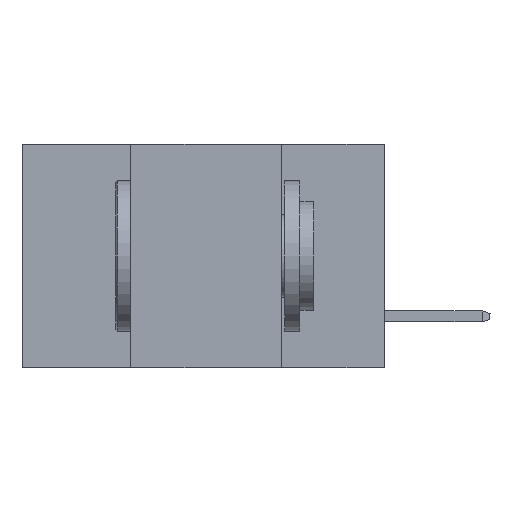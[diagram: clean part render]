
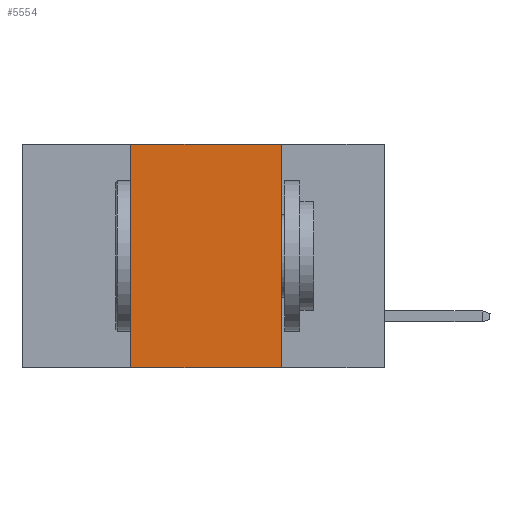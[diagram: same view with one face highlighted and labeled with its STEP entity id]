
A CAD part, left-side view. The second image highlights one B-rep face of the part: STEP entity #5554.
In plain terms, the highlighted planar face has unit normal (-1, 0, 0).
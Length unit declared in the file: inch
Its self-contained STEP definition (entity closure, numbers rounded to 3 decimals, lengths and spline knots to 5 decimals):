
#119 = CARTESIAN_POINT ( 'NONE',  ( 0., 0.17, 0. ) ) ;
#517 = VECTOR ( 'NONE', #2642, 39.37008 ) ;
#700 = DIRECTION ( 'NONE',  ( 0., -1., 0. ) ) ;
#762 = DIRECTION ( 'NONE',  ( 0., 0., -1. ) ) ;
#1027 = ORIENTED_EDGE ( 'NONE', *, *, #10004, .T. ) ;
#1449 = ORIENTED_EDGE ( 'NONE', *, *, #20818, .F. ) ;
#1867 = ORIENTED_EDGE ( 'NONE', *, *, #14197, .F. ) ;
#2285 = CARTESIAN_POINT ( 'NONE',  ( 0., 0.17, -0.37 ) ) ;
#2642 = DIRECTION ( 'NONE',  ( 0., 0., 1. ) ) ;
#2857 = LINE ( 'NONE', #10920, #517 ) ;
#3102 = VECTOR ( 'NONE', #15820, 39.37008 ) ;
#3290 = VERTEX_POINT ( 'NONE', #2285 ) ;
#3580 = DIRECTION ( 'NONE',  ( 1., 0., 0. ) ) ;
#4386 = VECTOR ( 'NONE', #700, 39.37008 ) ;
#5554 = ADVANCED_FACE ( 'NONE', ( #11743 ), #20213, .F. ) ;
#7330 = CARTESIAN_POINT ( 'NONE',  ( 0., 0.6, -0.37 ) ) ;
#8270 = EDGE_CURVE ( 'NONE', #14796, #3290, #19157, .T. ) ;
#9048 = LINE ( 'NONE', #7330, #18968 ) ;
#10004 = EDGE_CURVE ( 'NONE', #20821, #3290, #9048, .T. ) ;
#10497 = LINE ( 'NONE', #15432, #4386 ) ;
#10625 = CARTESIAN_POINT ( 'NONE',  ( 0., 0.42, 0. ) ) ;
#10920 = CARTESIAN_POINT ( 'NONE',  ( 0., 0.42, -0.37 ) ) ;
#11743 = FACE_OUTER_BOUND ( 'NONE', #13374, .T. ) ;
#11951 = AXIS2_PLACEMENT_3D ( 'NONE', #18276, #3580, #762 ) ;
#12623 = CARTESIAN_POINT ( 'NONE',  ( 0., 0.42, -0.37 ) ) ;
#13374 = EDGE_LOOP ( 'NONE', ( #16656, #1867, #1449, #1027 ) ) ;
#13596 = VERTEX_POINT ( 'NONE', #10625 ) ;
#14197 = EDGE_CURVE ( 'NONE', #13596, #14796, #10497, .T. ) ;
#14796 = VERTEX_POINT ( 'NONE', #119 ) ;
#15432 = CARTESIAN_POINT ( 'NONE',  ( 0., 0.6, 0. ) ) ;
#15820 = DIRECTION ( 'NONE',  ( 0., 0., -1. ) ) ;
#16656 = ORIENTED_EDGE ( 'NONE', *, *, #8270, .F. ) ;
#17731 = CARTESIAN_POINT ( 'NONE',  ( 0., 0.17, -0.37 ) ) ;
#18276 = CARTESIAN_POINT ( 'NONE',  ( 0., 0.6, 0. ) ) ;
#18905 = DIRECTION ( 'NONE',  ( 0., -1., 0. ) ) ;
#18968 = VECTOR ( 'NONE', #18905, 39.37008 ) ;
#19157 = LINE ( 'NONE', #17731, #3102 ) ;
#20213 = PLANE ( 'NONE',  #11951 ) ;
#20818 = EDGE_CURVE ( 'NONE', #20821, #13596, #2857, .T. ) ;
#20821 = VERTEX_POINT ( 'NONE', #12623 ) ;
